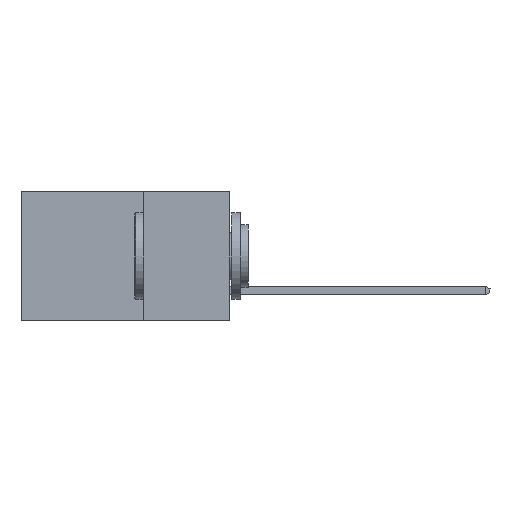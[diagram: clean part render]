
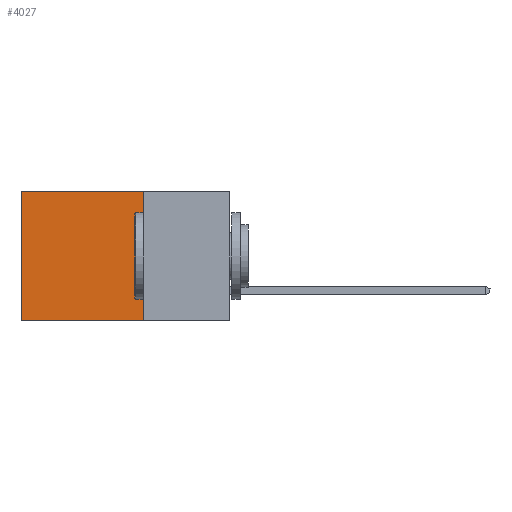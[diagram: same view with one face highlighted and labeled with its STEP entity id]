
A CAD part, left-side view. The second image highlights one B-rep face of the part: STEP entity #4027.
In plain terms, the highlighted planar face has unit normal (-1, 0, 0).
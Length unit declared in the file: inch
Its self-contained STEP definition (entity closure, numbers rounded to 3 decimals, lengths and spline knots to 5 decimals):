
#48 = EDGE_CURVE ( 'NONE', #12891, #5175, #12824, .T. ) ;
#698 = LINE ( 'NONE', #12957, #8582 ) ;
#742 = CARTESIAN_POINT ( 'NONE',  ( 0.2615, 0.6, -0.37 ) ) ;
#881 = ORIENTED_EDGE ( 'NONE', *, *, #3717, .T. ) ;
#2539 = LINE ( 'NONE', #17126, #15509 ) ;
#2609 = CARTESIAN_POINT ( 'NONE',  ( 0.2615, 0.6, -0.37 ) ) ;
#3213 = CARTESIAN_POINT ( 'NONE',  ( 0.2615, 0.25, 0. ) ) ;
#3585 = ORIENTED_EDGE ( 'NONE', *, *, #48, .T. ) ;
#3717 = EDGE_CURVE ( 'NONE', #13822, #12891, #2539, .T. ) ;
#3823 = DIRECTION ( 'NONE',  ( 0., 1., 0. ) ) ;
#3979 = VECTOR ( 'NONE', #5279, 39.37008 ) ;
#4027 = ADVANCED_FACE ( 'NONE', ( #15514 ), #4781, .F. ) ;
#4781 = PLANE ( 'NONE',  #6958 ) ;
#4838 = ORIENTED_EDGE ( 'NONE', *, *, #12263, .F. ) ;
#5175 = VERTEX_POINT ( 'NONE', #2609 ) ;
#5279 = DIRECTION ( 'NONE',  ( 0., 1., 0. ) ) ;
#5361 = LINE ( 'NONE', #12167, #3979 ) ;
#6148 = DIRECTION ( 'NONE',  ( 0., 0., -1. ) ) ;
#6958 = AXIS2_PLACEMENT_3D ( 'NONE', #8530, #12920, #8629 ) ;
#7629 = CARTESIAN_POINT ( 'NONE',  ( 0.2615, 0.6, 0. ) ) ;
#7793 = CARTESIAN_POINT ( 'NONE',  ( 0.2615, 0.25, -0.37 ) ) ;
#8530 = CARTESIAN_POINT ( 'NONE',  ( 0.2615, 0.25, -0.37 ) ) ;
#8582 = VECTOR ( 'NONE', #6148, 39.37008 ) ;
#8629 = DIRECTION ( 'NONE',  ( 0., 0., -1. ) ) ;
#10692 = VECTOR ( 'NONE', #15857, 39.37008 ) ;
#12167 = CARTESIAN_POINT ( 'NONE',  ( 0.2615, 0.25, -0.37 ) ) ;
#12263 = EDGE_CURVE ( 'NONE', #14787, #5175, #5361, .T. ) ;
#12824 = LINE ( 'NONE', #742, #10692 ) ;
#12891 = VERTEX_POINT ( 'NONE', #7629 ) ;
#12920 = DIRECTION ( 'NONE',  ( 1., 0., 0. ) ) ;
#12957 = CARTESIAN_POINT ( 'NONE',  ( 0.2615, 0.25, -0.37 ) ) ;
#13822 = VERTEX_POINT ( 'NONE', #3213 ) ;
#13863 = EDGE_CURVE ( 'NONE', #13822, #14787, #698, .T. ) ;
#14787 = VERTEX_POINT ( 'NONE', #7793 ) ;
#15056 = ORIENTED_EDGE ( 'NONE', *, *, #13863, .F. ) ;
#15117 = EDGE_LOOP ( 'NONE', ( #3585, #4838, #15056, #881 ) ) ;
#15509 = VECTOR ( 'NONE', #3823, 39.37008 ) ;
#15514 = FACE_OUTER_BOUND ( 'NONE', #15117, .T. ) ;
#15857 = DIRECTION ( 'NONE',  ( 0., 0., -1. ) ) ;
#17126 = CARTESIAN_POINT ( 'NONE',  ( 0.2615, 0.25, 0. ) ) ;
